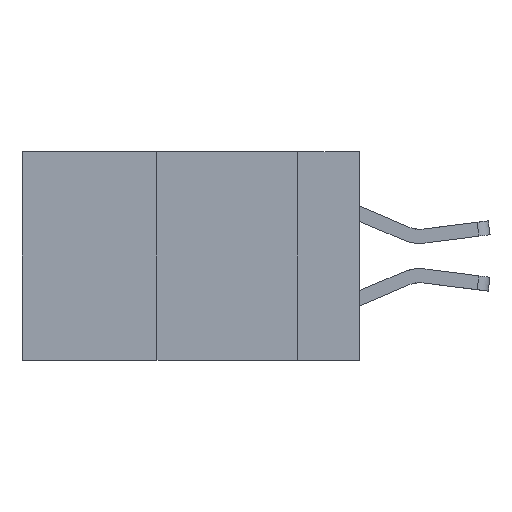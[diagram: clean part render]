
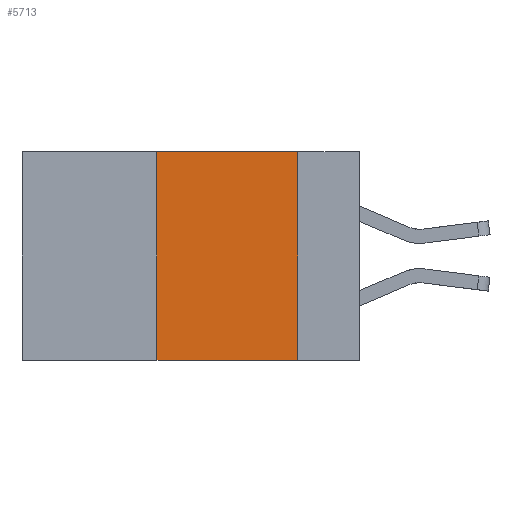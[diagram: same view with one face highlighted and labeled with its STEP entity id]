
A CAD part, left-side view. The second image highlights one B-rep face of the part: STEP entity #5713.
In plain terms, the highlighted planar face has unit normal (-1, 0, 0).
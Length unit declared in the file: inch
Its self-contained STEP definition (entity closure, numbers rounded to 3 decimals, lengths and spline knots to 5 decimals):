
#400 = VERTEX_POINT ( 'NONE', #2830 ) ;
#488 = EDGE_CURVE ( 'NONE', #2993, #400, #10784, .T. ) ;
#858 = DIRECTION ( 'NONE',  ( 0., 0., -1. ) ) ;
#2361 = CARTESIAN_POINT ( 'NONE',  ( 0., 0.6, 0. ) ) ;
#2399 = VECTOR ( 'NONE', #3954, 39.37008 ) ;
#2830 = CARTESIAN_POINT ( 'NONE',  ( 0., 0.11, -0.37 ) ) ;
#2993 = VERTEX_POINT ( 'NONE', #11553 ) ;
#3719 = VERTEX_POINT ( 'NONE', #5498 ) ;
#3738 = ORIENTED_EDGE ( 'NONE', *, *, #488, .F. ) ;
#3954 = DIRECTION ( 'NONE',  ( 0., -1., 0. ) ) ;
#4449 = DIRECTION ( 'NONE',  ( 0., 0., -1. ) ) ;
#4696 = EDGE_CURVE ( 'NONE', #3719, #400, #13095, .T. ) ;
#4714 = DIRECTION ( 'NONE',  ( 0., 0., 1. ) ) ;
#5498 = CARTESIAN_POINT ( 'NONE',  ( 0., 0.36, -0.37 ) ) ;
#5713 = ADVANCED_FACE ( 'NONE', ( #6917 ), #9560, .F. ) ;
#5863 = CARTESIAN_POINT ( 'NONE',  ( 0., 0.36, 0. ) ) ;
#6031 = DIRECTION ( 'NONE',  ( 0., -1., 0. ) ) ;
#6708 = VECTOR ( 'NONE', #6031, 39.37008 ) ;
#6810 = CARTESIAN_POINT ( 'NONE',  ( 0., 0.36, 0. ) ) ;
#6917 = FACE_OUTER_BOUND ( 'NONE', #12359, .T. ) ;
#7047 = LINE ( 'NONE', #12964, #6708 ) ;
#7176 = ORIENTED_EDGE ( 'NONE', *, *, #8071, .F. ) ;
#8071 = EDGE_CURVE ( 'NONE', #10549, #2993, #7047, .T. ) ;
#8163 = VECTOR ( 'NONE', #858, 39.37008 ) ;
#9050 = CARTESIAN_POINT ( 'NONE',  ( 0., 0.6, -0.37 ) ) ;
#9380 = LINE ( 'NONE', #6810, #11976 ) ;
#9388 = CARTESIAN_POINT ( 'NONE',  ( 0., 0.11, 0. ) ) ;
#9560 = PLANE ( 'NONE',  #10681 ) ;
#9761 = EDGE_CURVE ( 'NONE', #3719, #10549, #9380, .T. ) ;
#10528 = DIRECTION ( 'NONE',  ( 1., 0., 0. ) ) ;
#10549 = VERTEX_POINT ( 'NONE', #5863 ) ;
#10681 = AXIS2_PLACEMENT_3D ( 'NONE', #2361, #10528, #4449 ) ;
#10784 = LINE ( 'NONE', #9388, #8163 ) ;
#11044 = ORIENTED_EDGE ( 'NONE', *, *, #9761, .F. ) ;
#11553 = CARTESIAN_POINT ( 'NONE',  ( 0., 0.11, 0. ) ) ;
#11724 = ORIENTED_EDGE ( 'NONE', *, *, #4696, .T. ) ;
#11976 = VECTOR ( 'NONE', #4714, 39.37008 ) ;
#12359 = EDGE_LOOP ( 'NONE', ( #3738, #7176, #11044, #11724 ) ) ;
#12964 = CARTESIAN_POINT ( 'NONE',  ( 0., 0.6, 0. ) ) ;
#13095 = LINE ( 'NONE', #9050, #2399 ) ;
